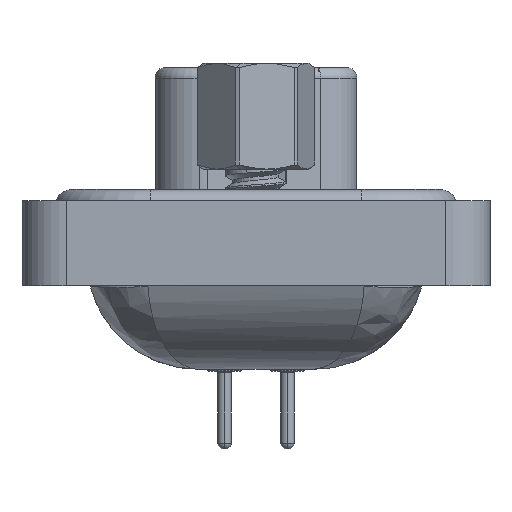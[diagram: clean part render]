
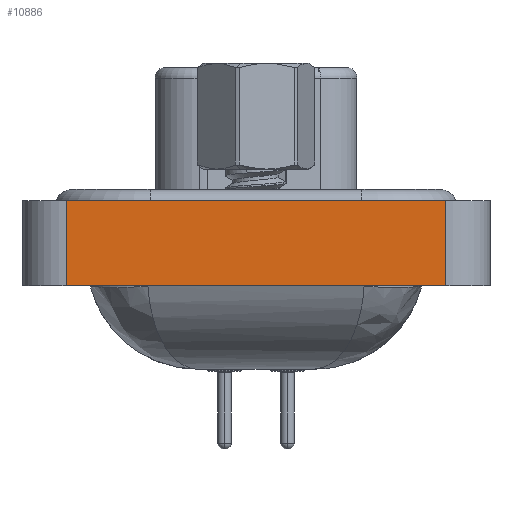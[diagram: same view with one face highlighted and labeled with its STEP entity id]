
A CAD part, left-side view. The second image highlights one B-rep face of the part: STEP entity #10886.
In plain terms, the highlighted planar face has unit normal (-1, 0, 0).
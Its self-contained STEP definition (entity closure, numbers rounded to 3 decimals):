
#461 = AXIS2_PLACEMENT_3D ( 'NONE', #11364, #16681, #6017 ) ;
#1737 = CARTESIAN_POINT ( 'NONE',  ( -7.15, 8.55, -3.35 ) ) ;
#1738 = DIRECTION ( 'NONE',  ( 0., -1., 0. ) ) ;
#2135 = VERTEX_POINT ( 'NONE', #20036 ) ;
#2650 = EDGE_CURVE ( 'NONE', #20904, #29919, #5467, .T. ) ;
#3117 = CARTESIAN_POINT ( 'NONE',  ( -7.15, 8.55, -3.35 ) ) ;
#5288 = EDGE_CURVE ( 'NONE', #20904, #5723, #22135, .T. ) ;
#5467 = LINE ( 'NONE', #3117, #23552 ) ;
#5687 = VECTOR ( 'NONE', #9625, 1000. ) ;
#5723 = VERTEX_POINT ( 'NONE', #14244 ) ;
#6017 = DIRECTION ( 'NONE',  ( 0., 0., 1. ) ) ;
#9462 = CARTESIAN_POINT ( 'NONE',  ( -7.15, -8.55, -3.35 ) ) ;
#9625 = DIRECTION ( 'NONE',  ( 0., 0., 1. ) ) ;
#10649 = DIRECTION ( 'NONE',  ( 0., 0., 1. ) ) ;
#10744 = EDGE_CURVE ( 'NONE', #29919, #2135, #20561, .T. ) ;
#10745 = ORIENTED_EDGE ( 'NONE', *, *, #10744, .F. ) ;
#10886 = ADVANCED_FACE ( 'NONE', ( #26242 ), #18693, .T. ) ;
#11364 = CARTESIAN_POINT ( 'NONE',  ( -7.15, -8.55, -3.35 ) ) ;
#13218 = DIRECTION ( 'NONE',  ( 0., -1., 0. ) ) ;
#13287 = EDGE_CURVE ( 'NONE', #5723, #2135, #19296, .T. ) ;
#14244 = CARTESIAN_POINT ( 'NONE',  ( -7.15, -8.55, -3.35 ) ) ;
#16681 = DIRECTION ( 'NONE',  ( -1., 0., 0. ) ) ;
#18693 = PLANE ( 'NONE',  #461 ) ;
#19020 = EDGE_LOOP ( 'NONE', ( #31293, #10745, #31079, #27106 ) ) ;
#19296 = LINE ( 'NONE', #9462, #5687 ) ;
#20036 = CARTESIAN_POINT ( 'NONE',  ( -7.15, -8.55, 0.5 ) ) ;
#20561 = LINE ( 'NONE', #28273, #23954 ) ;
#20904 = VERTEX_POINT ( 'NONE', #1737 ) ;
#22135 = LINE ( 'NONE', #32021, #32962 ) ;
#23552 = VECTOR ( 'NONE', #10649, 1000. ) ;
#23954 = VECTOR ( 'NONE', #13218, 1000. ) ;
#26242 = FACE_OUTER_BOUND ( 'NONE', #19020, .T. ) ;
#27106 = ORIENTED_EDGE ( 'NONE', *, *, #5288, .T. ) ;
#28273 = CARTESIAN_POINT ( 'NONE',  ( -7.15, -8.55, 0.5 ) ) ;
#28426 = CARTESIAN_POINT ( 'NONE',  ( -7.15, 8.55, 0.5 ) ) ;
#29919 = VERTEX_POINT ( 'NONE', #28426 ) ;
#31079 = ORIENTED_EDGE ( 'NONE', *, *, #2650, .F. ) ;
#31293 = ORIENTED_EDGE ( 'NONE', *, *, #13287, .T. ) ;
#32021 = CARTESIAN_POINT ( 'NONE',  ( -7.15, -8.55, -3.35 ) ) ;
#32962 = VECTOR ( 'NONE', #1738, 1000. ) ;
